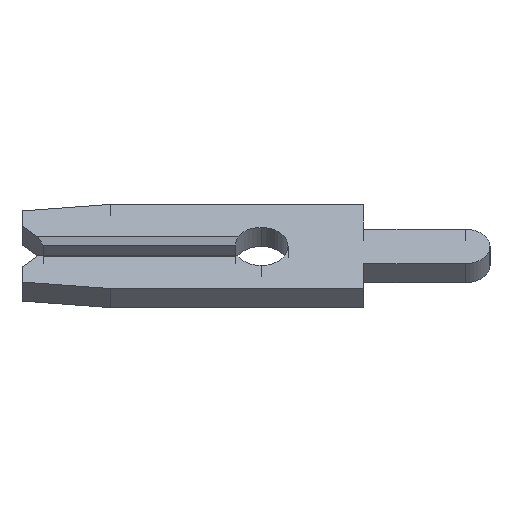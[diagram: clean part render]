
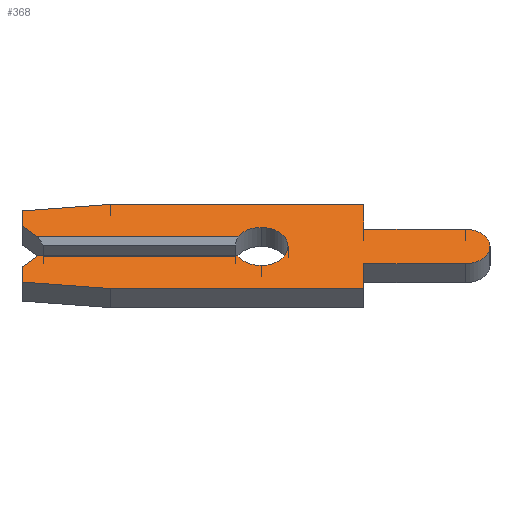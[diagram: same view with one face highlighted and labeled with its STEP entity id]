
A CAD part, left-side view. The second image highlights one B-rep face of the part: STEP entity #368.
In plain terms, the highlighted face is planar.
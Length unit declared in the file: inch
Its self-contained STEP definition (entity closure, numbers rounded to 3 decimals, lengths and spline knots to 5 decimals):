
#2 = CARTESIAN_POINT ( 'NONE',  ( -0.013, 0.146, 0.0575 ) ) ;
#10 = CARTESIAN_POINT ( 'NONE',  ( -0.013, 0.231, 0.04857 ) ) ;
#18 = EDGE_LOOP ( 'NONE', ( #1340, #767, #1550, #984, #1376, #443, #37, #1222, #20, #1786, #242, #1684, #720, #1741, #199, #485, #1722, #832 ) ) ;
#20 = ORIENTED_EDGE ( 'NONE', *, *, #1326, .F. ) ;
#26 = CARTESIAN_POINT ( 'NONE',  ( -0.013, 0.231, -0.028 ) ) ;
#32 = CARTESIAN_POINT ( 'NONE',  ( -0.013, -0.099, -0.0235 ) ) ;
#37 = ORIENTED_EDGE ( 'NONE', *, *, #1500, .F. ) ;
#48 = DIRECTION ( 'NONE',  ( 0., -0.707, 0.707 ) ) ;
#53 = VERTEX_POINT ( 'NONE', #873 ) ;
#68 = VERTEX_POINT ( 'NONE', #572 ) ;
#73 = CARTESIAN_POINT ( 'NONE',  ( -0.013, 0., 0. ) ) ;
#89 = LINE ( 'NONE', #1432, #131 ) ;
#113 = VECTOR ( 'NONE', #155, 39.37008 ) ;
#125 = CARTESIAN_POINT ( 'NONE',  ( -0.013, 0., 0. ) ) ;
#128 = VECTOR ( 'NONE', #364, 39.37008 ) ;
#131 = VECTOR ( 'NONE', #985, 39.37008 ) ;
#155 = DIRECTION ( 'NONE',  ( 0., 1., 0. ) ) ;
#157 = LINE ( 'NONE', #1760, #1220 ) ;
#172 = LINE ( 'NONE', #1661, #961 ) ;
#189 = CARTESIAN_POINT ( 'NONE',  ( -0.013, 0.231, 0.028 ) ) ;
#199 = ORIENTED_EDGE ( 'NONE', *, *, #511, .F. ) ;
#208 = CARTESIAN_POINT ( 'NONE',  ( -0.013, -0.1975, 0.0235 ) ) ;
#210 = LINE ( 'NONE', #1828, #128 ) ;
#219 = EDGE_CURVE ( 'NONE', #409, #1634, #1174, .T. ) ;
#242 = ORIENTED_EDGE ( 'NONE', *, *, #439, .F. ) ;
#244 = CARTESIAN_POINT ( 'NONE',  ( -0.013, 0., -0.013 ) ) ;
#251 = CARTESIAN_POINT ( 'NONE',  ( -0.013, 0.231, -0.04857 ) ) ;
#287 = DIRECTION ( 'NONE',  ( 1., 0., 0. ) ) ;
#289 = EDGE_CURVE ( 'NONE', #1634, #1059, #460, .T. ) ;
#306 = CARTESIAN_POINT ( 'NONE',  ( -0.013, -0.099, -0.0235 ) ) ;
#310 = LINE ( 'NONE', #558, #716 ) ;
#317 = VERTEX_POINT ( 'NONE', #2 ) ;
#335 = DIRECTION ( 'NONE',  ( 0., 0., 1. ) ) ;
#340 = VERTEX_POINT ( 'NONE', #26 ) ;
#360 = EDGE_CURVE ( 'NONE', #1606, #1805, #530, .T. ) ;
#364 = DIRECTION ( 'NONE',  ( 0., 0.995, 0.105 ) ) ;
#368 = ADVANCED_FACE ( 'NONE', ( #1339 ), #446, .F. ) ;
#402 = EDGE_CURVE ( 'NONE', #1128, #53, #157, .T. ) ;
#409 = VERTEX_POINT ( 'NONE', #1323 ) ;
#421 = DIRECTION ( 'NONE',  ( 0., 0., -1. ) ) ;
#431 = LINE ( 'NONE', #1037, #648 ) ;
#437 = DIRECTION ( 'NONE',  ( 0., 0., -1. ) ) ;
#439 = EDGE_CURVE ( 'NONE', #1059, #632, #1409, .T. ) ;
#443 = ORIENTED_EDGE ( 'NONE', *, *, #1373, .F. ) ;
#446 = PLANE ( 'NONE',  #1349 ) ;
#460 = CIRCLE ( 'NONE', #704, 0.0235 ) ;
#467 = CARTESIAN_POINT ( 'NONE',  ( -0.013, -0.1975, 0. ) ) ;
#485 = ORIENTED_EDGE ( 'NONE', *, *, #833, .F. ) ;
#511 = EDGE_CURVE ( 'NONE', #317, #902, #1295, .T. ) ;
#516 = CARTESIAN_POINT ( 'NONE',  ( -0.013, 0.216, -0.013 ) ) ;
#530 = CIRCLE ( 'NONE', #1192, 0.026 ) ;
#558 = CARTESIAN_POINT ( 'NONE',  ( -0.013, -0.099, -0.0575 ) ) ;
#572 = CARTESIAN_POINT ( 'NONE',  ( -0.013, 0.146, -0.0575 ) ) ;
#602 = DIRECTION ( 'NONE',  ( 0., 1., 0. ) ) ;
#609 = EDGE_CURVE ( 'NONE', #1524, #1366, #876, .T. ) ;
#610 = CARTESIAN_POINT ( 'NONE',  ( -0.013, 0., 0. ) ) ;
#614 = CARTESIAN_POINT ( 'NONE',  ( -0.013, 0.2105, -0.0075 ) ) ;
#616 = DIRECTION ( 'NONE',  ( 0., -1., 0. ) ) ;
#627 = VECTOR ( 'NONE', #1490, 39.37008 ) ;
#632 = VERTEX_POINT ( 'NONE', #32 ) ;
#638 = DIRECTION ( 'NONE',  ( 0., -1., 0. ) ) ;
#644 = CARTESIAN_POINT ( 'NONE',  ( -0.013, 0.2105, 0.0075 ) ) ;
#648 = VECTOR ( 'NONE', #602, 39.37008 ) ;
#652 = DIRECTION ( 'NONE',  ( 0., 0.707, 0.707 ) ) ;
#658 = CARTESIAN_POINT ( 'NONE',  ( -0.013, -0.099, -0.0575 ) ) ;
#694 = VECTOR ( 'NONE', #638, 39.37008 ) ;
#704 = AXIS2_PLACEMENT_3D ( 'NONE', #467, #1479, #749 ) ;
#713 = VECTOR ( 'NONE', #652, 39.37008 ) ;
#716 = VECTOR ( 'NONE', #437, 39.37008 ) ;
#720 = ORIENTED_EDGE ( 'NONE', *, *, #219, .F. ) ;
#749 = DIRECTION ( 'NONE',  ( 0., 0., 1. ) ) ;
#767 = ORIENTED_EDGE ( 'NONE', *, *, #1058, .F. ) ;
#823 = VECTOR ( 'NONE', #1145, 39.37008 ) ;
#832 = ORIENTED_EDGE ( 'NONE', *, *, #1526, .F. ) ;
#833 = EDGE_CURVE ( 'NONE', #1366, #317, #89, .T. ) ;
#873 = CARTESIAN_POINT ( 'NONE',  ( -0.013, 0.02252, 0.013 ) ) ;
#876 = LINE ( 'NONE', #1204, #1658 ) ;
#878 = VERTEX_POINT ( 'NONE', #658 ) ;
#902 = VERTEX_POINT ( 'NONE', #1822 ) ;
#945 = VECTOR ( 'NONE', #1265, 39.37008 ) ;
#961 = VECTOR ( 'NONE', #335, 39.37008 ) ;
#984 = ORIENTED_EDGE ( 'NONE', *, *, #1810, .F. ) ;
#985 = DIRECTION ( 'NONE',  ( 0., -0.995, 0.105 ) ) ;
#1037 = CARTESIAN_POINT ( 'NONE',  ( -0.013, 0.146, -0.0575 ) ) ;
#1058 = EDGE_CURVE ( 'NONE', #1805, #53, #1425, .T. ) ;
#1059 = VERTEX_POINT ( 'NONE', #1436 ) ;
#1062 = EDGE_CURVE ( 'NONE', #1102, #1382, #1655, .T. ) ;
#1063 = DIRECTION ( 'NONE',  ( 0., 0., 1. ) ) ;
#1084 = VERTEX_POINT ( 'NONE', #251 ) ;
#1096 = EDGE_CURVE ( 'NONE', #632, #878, #310, .T. ) ;
#1102 = VERTEX_POINT ( 'NONE', #516 ) ;
#1128 = VERTEX_POINT ( 'NONE', #1751 ) ;
#1145 = DIRECTION ( 'NONE',  ( 0., -1., 0. ) ) ;
#1174 = LINE ( 'NONE', #1341, #627 ) ;
#1175 = CARTESIAN_POINT ( 'NONE',  ( -0.013, 0., 0. ) ) ;
#1192 = AXIS2_PLACEMENT_3D ( 'NONE', #1175, #1483, #1198 ) ;
#1198 = DIRECTION ( 'NONE',  ( 0., 0., -1. ) ) ;
#1204 = CARTESIAN_POINT ( 'NONE',  ( -0.013, 0.231, 0.028 ) ) ;
#1212 = DIRECTION ( 'NONE',  ( -1., 0., 0. ) ) ;
#1215 = LINE ( 'NONE', #644, #713 ) ;
#1220 = VECTOR ( 'NONE', #616, 39.37008 ) ;
#1222 = ORIENTED_EDGE ( 'NONE', *, *, #1807, .F. ) ;
#1242 = CIRCLE ( 'NONE', #1657, 0.026 ) ;
#1248 = CARTESIAN_POINT ( 'NONE',  ( -0.013, 0., 0.026 ) ) ;
#1254 = DIRECTION ( 'NONE',  ( -1., 0., 0. ) ) ;
#1265 = DIRECTION ( 'NONE',  ( 0., 0., -1. ) ) ;
#1295 = LINE ( 'NONE', #1650, #694 ) ;
#1313 = VECTOR ( 'NONE', #48, 39.37008 ) ;
#1323 = CARTESIAN_POINT ( 'NONE',  ( -0.013, -0.099, 0.0235 ) ) ;
#1326 = EDGE_CURVE ( 'NONE', #878, #68, #431, .T. ) ;
#1338 = LINE ( 'NONE', #1403, #945 ) ;
#1339 = FACE_OUTER_BOUND ( 'NONE', #18, .T. ) ;
#1340 = ORIENTED_EDGE ( 'NONE', *, *, #402, .T. ) ;
#1341 = CARTESIAN_POINT ( 'NONE',  ( -0.013, -0.099, 0.0235 ) ) ;
#1349 = AXIS2_PLACEMENT_3D ( 'NONE', #610, #287, #1626 ) ;
#1366 = VERTEX_POINT ( 'NONE', #10 ) ;
#1368 = CARTESIAN_POINT ( 'NONE',  ( -0.013, 0., -0.026 ) ) ;
#1373 = EDGE_CURVE ( 'NONE', #340, #1102, #1757, .T. ) ;
#1376 = ORIENTED_EDGE ( 'NONE', *, *, #1062, .F. ) ;
#1379 = CARTESIAN_POINT ( 'NONE',  ( -0.013, 0.02252, -0.013 ) ) ;
#1382 = VERTEX_POINT ( 'NONE', #1379 ) ;
#1403 = CARTESIAN_POINT ( 'NONE',  ( -0.013, -0.099, 0.0575 ) ) ;
#1409 = LINE ( 'NONE', #306, #113 ) ;
#1425 = CIRCLE ( 'NONE', #1651, 0.026 ) ;
#1432 = CARTESIAN_POINT ( 'NONE',  ( -0.013, 0.231, 0.04857 ) ) ;
#1436 = CARTESIAN_POINT ( 'NONE',  ( -0.013, -0.1975, -0.0235 ) ) ;
#1479 = DIRECTION ( 'NONE',  ( 1., 0., 0. ) ) ;
#1483 = DIRECTION ( 'NONE',  ( -1., 0., 0. ) ) ;
#1490 = DIRECTION ( 'NONE',  ( 0., -1., 0. ) ) ;
#1500 = EDGE_CURVE ( 'NONE', #1084, #340, #172, .T. ) ;
#1524 = VERTEX_POINT ( 'NONE', #189 ) ;
#1526 = EDGE_CURVE ( 'NONE', #1128, #1524, #1215, .T. ) ;
#1545 = DIRECTION ( 'NONE',  ( 0., 0., -1. ) ) ;
#1550 = ORIENTED_EDGE ( 'NONE', *, *, #360, .F. ) ;
#1606 = VERTEX_POINT ( 'NONE', #1368 ) ;
#1626 = DIRECTION ( 'NONE',  ( 0., 0., -1. ) ) ;
#1634 = VERTEX_POINT ( 'NONE', #208 ) ;
#1650 = CARTESIAN_POINT ( 'NONE',  ( -0.013, 0.146, 0.0575 ) ) ;
#1651 = AXIS2_PLACEMENT_3D ( 'NONE', #125, #1212, #421 ) ;
#1655 = LINE ( 'NONE', #244, #823 ) ;
#1657 = AXIS2_PLACEMENT_3D ( 'NONE', #73, #1254, #1545 ) ;
#1658 = VECTOR ( 'NONE', #1063, 39.37008 ) ;
#1661 = CARTESIAN_POINT ( 'NONE',  ( -0.013, 0.231, -0.028 ) ) ;
#1662 = EDGE_CURVE ( 'NONE', #902, #409, #1338, .T. ) ;
#1684 = ORIENTED_EDGE ( 'NONE', *, *, #289, .F. ) ;
#1722 = ORIENTED_EDGE ( 'NONE', *, *, #609, .F. ) ;
#1741 = ORIENTED_EDGE ( 'NONE', *, *, #1662, .F. ) ;
#1751 = CARTESIAN_POINT ( 'NONE',  ( -0.013, 0.216, 0.013 ) ) ;
#1757 = LINE ( 'NONE', #614, #1313 ) ;
#1760 = CARTESIAN_POINT ( 'NONE',  ( -0.013, 0.231, 0.013 ) ) ;
#1786 = ORIENTED_EDGE ( 'NONE', *, *, #1096, .F. ) ;
#1805 = VERTEX_POINT ( 'NONE', #1248 ) ;
#1807 = EDGE_CURVE ( 'NONE', #68, #1084, #210, .T. ) ;
#1810 = EDGE_CURVE ( 'NONE', #1382, #1606, #1242, .T. ) ;
#1822 = CARTESIAN_POINT ( 'NONE',  ( -0.013, -0.099, 0.0575 ) ) ;
#1828 = CARTESIAN_POINT ( 'NONE',  ( -0.013, 0.231, -0.04857 ) ) ;
